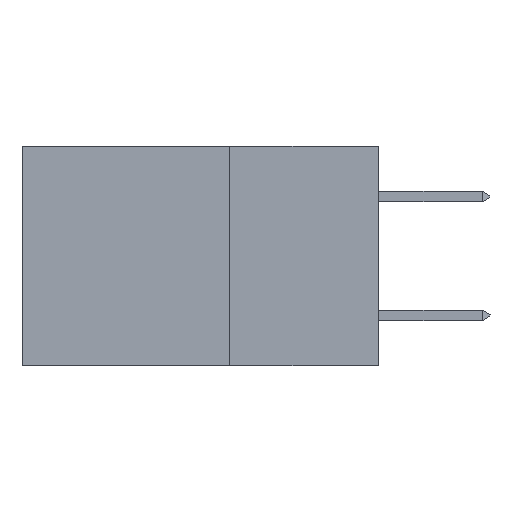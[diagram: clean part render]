
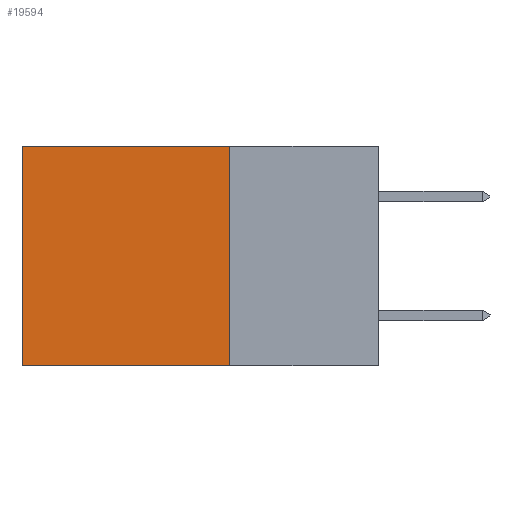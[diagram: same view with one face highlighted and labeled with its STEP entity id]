
A CAD part, left-side view. The second image highlights one B-rep face of the part: STEP entity #19594.
In plain terms, the highlighted planar face has unit normal (-1, 0, 0).
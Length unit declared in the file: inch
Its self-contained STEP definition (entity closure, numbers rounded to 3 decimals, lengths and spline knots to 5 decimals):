
#102 = CARTESIAN_POINT ( 'NONE',  ( 0.298, 0.25, -0.37 ) ) ;
#345 = CARTESIAN_POINT ( 'NONE',  ( 0.298, 0.25, 0. ) ) ;
#541 = EDGE_CURVE ( 'NONE', #9246, #738, #10418, .T. ) ;
#738 = VERTEX_POINT ( 'NONE', #102 ) ;
#1298 = VECTOR ( 'NONE', #6511, 39.37008 ) ;
#2880 = VECTOR ( 'NONE', #2903, 39.37008 ) ;
#2903 = DIRECTION ( 'NONE',  ( 0., 0., -1. ) ) ;
#4133 = DIRECTION ( 'NONE',  ( 1., 0., 0. ) ) ;
#5926 = CARTESIAN_POINT ( 'NONE',  ( 0.298, 0.25, 0. ) ) ;
#5939 = ORIENTED_EDGE ( 'NONE', *, *, #24723, .F. ) ;
#6189 = VERTEX_POINT ( 'NONE', #22660 ) ;
#6511 = DIRECTION ( 'NONE',  ( 0., 1., 0. ) ) ;
#7729 = EDGE_CURVE ( 'NONE', #6189, #13866, #8299, .T. ) ;
#8299 = LINE ( 'NONE', #8945, #2880 ) ;
#8945 = CARTESIAN_POINT ( 'NONE',  ( 0.298, 0.6, 0. ) ) ;
#9246 = VERTEX_POINT ( 'NONE', #11302 ) ;
#9976 = ORIENTED_EDGE ( 'NONE', *, *, #7729, .T. ) ;
#10135 = PLANE ( 'NONE',  #10353 ) ;
#10210 = CARTESIAN_POINT ( 'NONE',  ( 0.298, 0.6, -0.37 ) ) ;
#10353 = AXIS2_PLACEMENT_3D ( 'NONE', #16309, #4133, #18331 ) ;
#10418 = LINE ( 'NONE', #5926, #25177 ) ;
#11302 = CARTESIAN_POINT ( 'NONE',  ( 0.298, 0.25, 0. ) ) ;
#12511 = VECTOR ( 'NONE', #19888, 39.37008 ) ;
#13636 = ORIENTED_EDGE ( 'NONE', *, *, #19720, .T. ) ;
#13866 = VERTEX_POINT ( 'NONE', #10210 ) ;
#15532 = ORIENTED_EDGE ( 'NONE', *, *, #541, .F. ) ;
#16309 = CARTESIAN_POINT ( 'NONE',  ( 0.298, 0.25, 0. ) ) ;
#17537 = LINE ( 'NONE', #345, #1298 ) ;
#18331 = DIRECTION ( 'NONE',  ( 0., 0., -1. ) ) ;
#19594 = ADVANCED_FACE ( 'NONE', ( #25290 ), #10135, .F. ) ;
#19720 = EDGE_CURVE ( 'NONE', #9246, #6189, #17537, .T. ) ;
#19888 = DIRECTION ( 'NONE',  ( 0., 1., 0. ) ) ;
#21941 = CARTESIAN_POINT ( 'NONE',  ( 0.298, 0.25, -0.37 ) ) ;
#22550 = LINE ( 'NONE', #21941, #12511 ) ;
#22660 = CARTESIAN_POINT ( 'NONE',  ( 0.298, 0.6, 0. ) ) ;
#24204 = EDGE_LOOP ( 'NONE', ( #9976, #5939, #15532, #13636 ) ) ;
#24723 = EDGE_CURVE ( 'NONE', #738, #13866, #22550, .T. ) ;
#25177 = VECTOR ( 'NONE', #25361, 39.37008 ) ;
#25290 = FACE_OUTER_BOUND ( 'NONE', #24204, .T. ) ;
#25361 = DIRECTION ( 'NONE',  ( 0., 0., -1. ) ) ;
